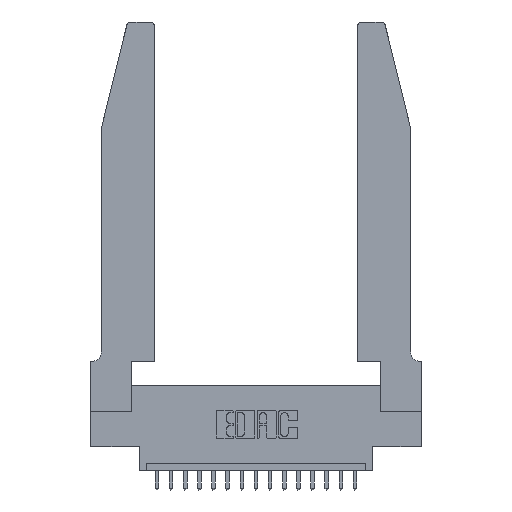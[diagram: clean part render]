
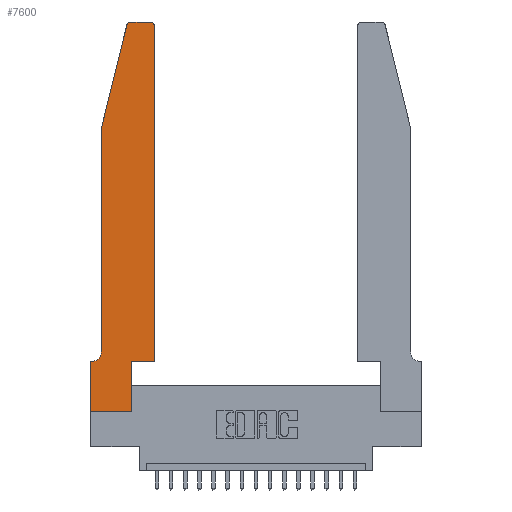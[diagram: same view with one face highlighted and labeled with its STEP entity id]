
A CAD part, top view. The second image highlights one B-rep face of the part: STEP entity #7600.
In plain terms, the highlighted planar face has unit normal (0, 0, 1).
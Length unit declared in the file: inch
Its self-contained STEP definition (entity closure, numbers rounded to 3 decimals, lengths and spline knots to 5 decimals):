
#116 = VECTOR ( 'NONE', #15611, 39.37008 ) ;
#136 = LINE ( 'NONE', #8082, #7338 ) ;
#611 = LINE ( 'NONE', #15677, #116 ) ;
#948 = CARTESIAN_POINT ( 'NONE',  ( 0.2865, 0., 0.37 ) ) ;
#957 = VECTOR ( 'NONE', #10759, 39.37008 ) ;
#981 = VERTEX_POINT ( 'NONE', #10108 ) ;
#1104 = EDGE_CURVE ( 'NONE', #981, #15567, #1878, .T. ) ;
#1125 = AXIS2_PLACEMENT_3D ( 'NONE', #13607, #17983, #7348 ) ;
#1411 = AXIS2_PLACEMENT_3D ( 'NONE', #5640, #4009, #3942 ) ;
#1552 = FACE_OUTER_BOUND ( 'NONE', #19493, .T. ) ;
#1878 = LINE ( 'NONE', #2637, #3803 ) ;
#2363 = VERTEX_POINT ( 'NONE', #5338 ) ;
#2399 = ORIENTED_EDGE ( 'NONE', *, *, #19187, .T. ) ;
#2637 = CARTESIAN_POINT ( 'NONE',  ( 0., 0., 0.37 ) ) ;
#3046 = CARTESIAN_POINT ( 'NONE',  ( 0.0755, 2., 0.37 ) ) ;
#3269 = ORIENTED_EDGE ( 'NONE', *, *, #17650, .T. ) ;
#3285 = DIRECTION ( 'NONE',  ( 0., 1., 0. ) ) ;
#3511 = EDGE_CURVE ( 'NONE', #9169, #12621, #136, .T. ) ;
#3642 = EDGE_CURVE ( 'NONE', #11098, #8048, #17641, .T. ) ;
#3675 = PLANE ( 'NONE',  #1411 ) ;
#3803 = VECTOR ( 'NONE', #13418, 39.37008 ) ;
#3910 = CIRCLE ( 'NONE', #12472, 0.03 ) ;
#3931 = LINE ( 'NONE', #8557, #5632 ) ;
#3942 = DIRECTION ( 'NONE',  ( 1., 0., 0. ) ) ;
#3988 = ORIENTED_EDGE ( 'NONE', *, *, #3511, .T. ) ;
#4009 = DIRECTION ( 'NONE',  ( 0., 0., 1. ) ) ;
#4374 = ORIENTED_EDGE ( 'NONE', *, *, #9426, .T. ) ;
#4677 = CIRCLE ( 'NONE', #1125, 0.07 ) ;
#4775 = CARTESIAN_POINT ( 'NONE',  ( 0.0055, 0.35, 0.37 ) ) ;
#4916 = LINE ( 'NONE', #13342, #14757 ) ;
#5066 = EDGE_CURVE ( 'NONE', #5737, #2363, #5532, .T. ) ;
#5338 = CARTESIAN_POINT ( 'NONE',  ( 0.2865, 0.35, 0.37 ) ) ;
#5532 = LINE ( 'NONE', #13502, #957 ) ;
#5558 = VERTEX_POINT ( 'NONE', #8713 ) ;
#5632 = VECTOR ( 'NONE', #11871, 39.37008 ) ;
#5640 = CARTESIAN_POINT ( 'NONE',  ( 0., 0.35, 0.37 ) ) ;
#5737 = VERTEX_POINT ( 'NONE', #948 ) ;
#5845 = CARTESIAN_POINT ( 'NONE',  ( 0.284, 2.75, 0.37 ) ) ;
#6380 = DIRECTION ( 'NONE',  ( 0., 0., 1. ) ) ;
#6886 = VERTEX_POINT ( 'NONE', #4775 ) ;
#7254 = LINE ( 'NONE', #9401, #10138 ) ;
#7338 = VECTOR ( 'NONE', #3285, 39.37008 ) ;
#7348 = DIRECTION ( 'NONE',  ( -1., 0., 0. ) ) ;
#7547 = EDGE_CURVE ( 'NONE', #5558, #13804, #4916, .T. ) ;
#7600 = ADVANCED_FACE ( 'NONE', ( #1552 ), #3675, .T. ) ;
#7667 = DIRECTION ( 'NONE',  ( 0., -1., 0. ) ) ;
#7948 = DIRECTION ( 'NONE',  ( 0., 0., 1. ) ) ;
#8015 = ORIENTED_EDGE ( 'NONE', *, *, #12909, .T. ) ;
#8048 = VERTEX_POINT ( 'NONE', #8124 ) ;
#8082 = CARTESIAN_POINT ( 'NONE',  ( 0.4505, 0.35, 0.37 ) ) ;
#8124 = CARTESIAN_POINT ( 'NONE',  ( 0.0755, 0.42, 0.37 ) ) ;
#8338 = LINE ( 'NONE', #15773, #13333 ) ;
#8557 = CARTESIAN_POINT ( 'NONE',  ( 0.0755, 2., 0.37 ) ) ;
#8642 = ORIENTED_EDGE ( 'NONE', *, *, #7547, .T. ) ;
#8713 = CARTESIAN_POINT ( 'NONE',  ( 0.4205, 2.75, 0.37 ) ) ;
#8738 = CARTESIAN_POINT ( 'NONE',  ( 0., 0., 0.37 ) ) ;
#9169 = VERTEX_POINT ( 'NONE', #17465 ) ;
#9401 = CARTESIAN_POINT ( 'NONE',  ( 0., 0., 0.37 ) ) ;
#9426 = EDGE_CURVE ( 'NONE', #13804, #13417, #10603, .T. ) ;
#9427 = EDGE_CURVE ( 'NONE', #12621, #5558, #3910, .T. ) ;
#9459 = DIRECTION ( 'NONE',  ( 1., 0., 0. ) ) ;
#9491 = VECTOR ( 'NONE', #7667, 39.37008 ) ;
#10108 = CARTESIAN_POINT ( 'NONE',  ( 0., 0.35, 0.37 ) ) ;
#10138 = VECTOR ( 'NONE', #9459, 39.37008 ) ;
#10603 = CIRCLE ( 'NONE', #11462, 0.03 ) ;
#10759 = DIRECTION ( 'NONE',  ( 0., 1., 0. ) ) ;
#11098 = VERTEX_POINT ( 'NONE', #3046 ) ;
#11462 = AXIS2_PLACEMENT_3D ( 'NONE', #15686, #7948, #13998 ) ;
#11647 = CARTESIAN_POINT ( 'NONE',  ( 0.25487, 2.72718, 0.37 ) ) ;
#11691 = CARTESIAN_POINT ( 'NONE',  ( 0.4505, 2.72, 0.37 ) ) ;
#11871 = DIRECTION ( 'NONE',  ( -0.239, -0.971, 0. ) ) ;
#12059 = EDGE_CURVE ( 'NONE', #13417, #11098, #3931, .T. ) ;
#12472 = AXIS2_PLACEMENT_3D ( 'NONE', #18633, #6380, #17095 ) ;
#12621 = VERTEX_POINT ( 'NONE', #11691 ) ;
#12909 = EDGE_CURVE ( 'NONE', #15567, #5737, #7254, .T. ) ;
#13012 = ORIENTED_EDGE ( 'NONE', *, *, #1104, .T. ) ;
#13255 = ORIENTED_EDGE ( 'NONE', *, *, #16758, .T. ) ;
#13333 = VECTOR ( 'NONE', #14150, 39.37008 ) ;
#13342 = CARTESIAN_POINT ( 'NONE',  ( 0.2605, 2.75, 0.37 ) ) ;
#13417 = VERTEX_POINT ( 'NONE', #11647 ) ;
#13418 = DIRECTION ( 'NONE',  ( 0., -1., 0. ) ) ;
#13502 = CARTESIAN_POINT ( 'NONE',  ( 0.2865, 0.35, 0.37 ) ) ;
#13607 = CARTESIAN_POINT ( 'NONE',  ( 0.0055, 0.42, 0.37 ) ) ;
#13804 = VERTEX_POINT ( 'NONE', #5845 ) ;
#13998 = DIRECTION ( 'NONE',  ( 1., 0., 0. ) ) ;
#14063 = ORIENTED_EDGE ( 'NONE', *, *, #12059, .T. ) ;
#14150 = DIRECTION ( 'NONE',  ( 1., 0., 0. ) ) ;
#14757 = VECTOR ( 'NONE', #19573, 39.37008 ) ;
#15041 = ORIENTED_EDGE ( 'NONE', *, *, #3642, .T. ) ;
#15567 = VERTEX_POINT ( 'NONE', #8738 ) ;
#15611 = DIRECTION ( 'NONE',  ( -1., 0., 0. ) ) ;
#15677 = CARTESIAN_POINT ( 'NONE',  ( 0.0755, 0.35, 0.37 ) ) ;
#15686 = CARTESIAN_POINT ( 'NONE',  ( 0.284, 2.72, 0.37 ) ) ;
#15773 = CARTESIAN_POINT ( 'NONE',  ( 0.4505, 0.35, 0.37 ) ) ;
#16758 = EDGE_CURVE ( 'NONE', #8048, #6886, #4677, .T. ) ;
#16821 = CARTESIAN_POINT ( 'NONE',  ( 0.0755, 2., 0.37 ) ) ;
#17095 = DIRECTION ( 'NONE',  ( 1., 0., 0. ) ) ;
#17465 = CARTESIAN_POINT ( 'NONE',  ( 0.4505, 0.35, 0.37 ) ) ;
#17641 = LINE ( 'NONE', #16821, #9491 ) ;
#17650 = EDGE_CURVE ( 'NONE', #2363, #9169, #8338, .T. ) ;
#17761 = ORIENTED_EDGE ( 'NONE', *, *, #9427, .T. ) ;
#17983 = DIRECTION ( 'NONE',  ( 0., 0., -1. ) ) ;
#18012 = ORIENTED_EDGE ( 'NONE', *, *, #5066, .T. ) ;
#18633 = CARTESIAN_POINT ( 'NONE',  ( 0.4205, 2.72, 0.37 ) ) ;
#19187 = EDGE_CURVE ( 'NONE', #6886, #981, #611, .T. ) ;
#19493 = EDGE_LOOP ( 'NONE', ( #8642, #4374, #14063, #15041, #13255, #2399, #13012, #8015, #18012, #3269, #3988, #17761 ) ) ;
#19573 = DIRECTION ( 'NONE',  ( -1., 0., 0. ) ) ;
